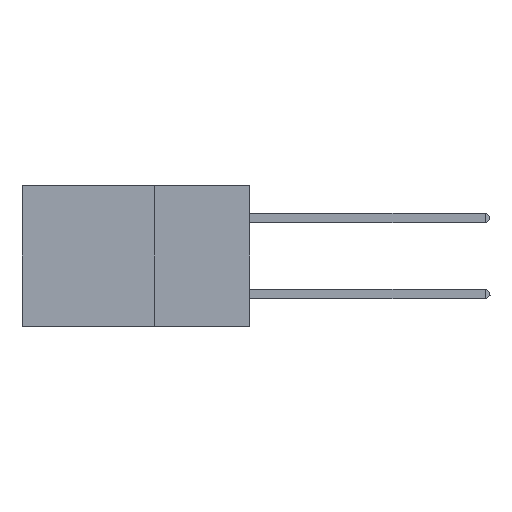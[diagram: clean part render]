
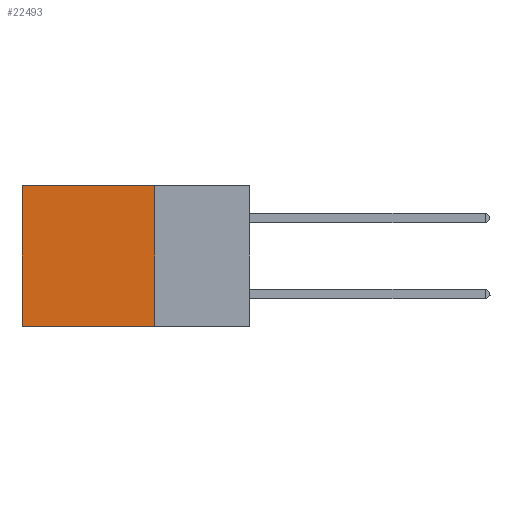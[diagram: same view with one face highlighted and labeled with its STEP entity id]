
A CAD part, left-side view. The second image highlights one B-rep face of the part: STEP entity #22493.
In plain terms, the highlighted planar face has unit normal (-1, 0, 0).
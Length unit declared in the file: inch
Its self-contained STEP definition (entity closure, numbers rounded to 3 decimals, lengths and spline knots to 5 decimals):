
#114 = VERTEX_POINT ( 'NONE', #2734 ) ;
#2019 = LINE ( 'NONE', #12569, #25348 ) ;
#2195 = DIRECTION ( 'NONE',  ( 1., 0., 0. ) ) ;
#2734 = CARTESIAN_POINT ( 'NONE',  ( 0.2875, 0.25, -0.37 ) ) ;
#7240 = FACE_OUTER_BOUND ( 'NONE', #33227, .T. ) ;
#7269 = ORIENTED_EDGE ( 'NONE', *, *, #33427, .T. ) ;
#8593 = ORIENTED_EDGE ( 'NONE', *, *, #22029, .F. ) ;
#8748 = VERTEX_POINT ( 'NONE', #25910 ) ;
#8973 = VERTEX_POINT ( 'NONE', #13800 ) ;
#12569 = CARTESIAN_POINT ( 'NONE',  ( 0.2875, 0.25, 0. ) ) ;
#12582 = ORIENTED_EDGE ( 'NONE', *, *, #36549, .F. ) ;
#13158 = AXIS2_PLACEMENT_3D ( 'NONE', #26924, #2195, #27689 ) ;
#13800 = CARTESIAN_POINT ( 'NONE',  ( 0.2875, 0.6, 0. ) ) ;
#14349 = ORIENTED_EDGE ( 'NONE', *, *, #39575, .T. ) ;
#14545 = CARTESIAN_POINT ( 'NONE',  ( 0.2875, 0.6, 0. ) ) ;
#17186 = LINE ( 'NONE', #27333, #23502 ) ;
#20232 = DIRECTION ( 'NONE',  ( 0., 1., 0. ) ) ;
#20705 = DIRECTION ( 'NONE',  ( 0., 1., 0. ) ) ;
#21178 = CARTESIAN_POINT ( 'NONE',  ( 0.2875, 0.25, -0.37 ) ) ;
#21649 = LINE ( 'NONE', #14545, #34711 ) ;
#22029 = EDGE_CURVE ( 'NONE', #114, #36185, #39285, .T. ) ;
#22493 = ADVANCED_FACE ( 'NONE', ( #7240 ), #22827, .F. ) ;
#22827 = PLANE ( 'NONE',  #13158 ) ;
#23502 = VECTOR ( 'NONE', #20705, 39.37008 ) ;
#25348 = VECTOR ( 'NONE', #38366, 39.37008 ) ;
#25910 = CARTESIAN_POINT ( 'NONE',  ( 0.2875, 0.25, 0. ) ) ;
#26627 = CARTESIAN_POINT ( 'NONE',  ( 0.2875, 0.6, -0.37 ) ) ;
#26924 = CARTESIAN_POINT ( 'NONE',  ( 0.2875, 0.25, 0. ) ) ;
#27333 = CARTESIAN_POINT ( 'NONE',  ( 0.2875, 0.25, 0. ) ) ;
#27689 = DIRECTION ( 'NONE',  ( 0., 0., -1. ) ) ;
#32826 = DIRECTION ( 'NONE',  ( 0., 0., -1. ) ) ;
#33227 = EDGE_LOOP ( 'NONE', ( #14349, #8593, #12582, #7269 ) ) ;
#33427 = EDGE_CURVE ( 'NONE', #8748, #8973, #17186, .T. ) ;
#34711 = VECTOR ( 'NONE', #32826, 39.37008 ) ;
#36185 = VERTEX_POINT ( 'NONE', #26627 ) ;
#36549 = EDGE_CURVE ( 'NONE', #8748, #114, #2019, .T. ) ;
#38292 = VECTOR ( 'NONE', #20232, 39.37008 ) ;
#38366 = DIRECTION ( 'NONE',  ( 0., 0., -1. ) ) ;
#39285 = LINE ( 'NONE', #21178, #38292 ) ;
#39575 = EDGE_CURVE ( 'NONE', #8973, #36185, #21649, .T. ) ;
